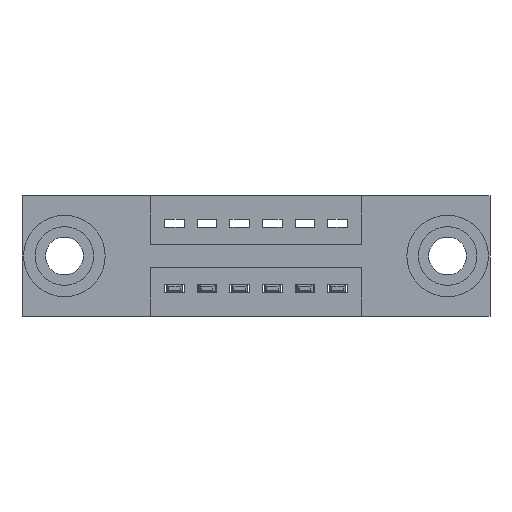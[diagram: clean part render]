
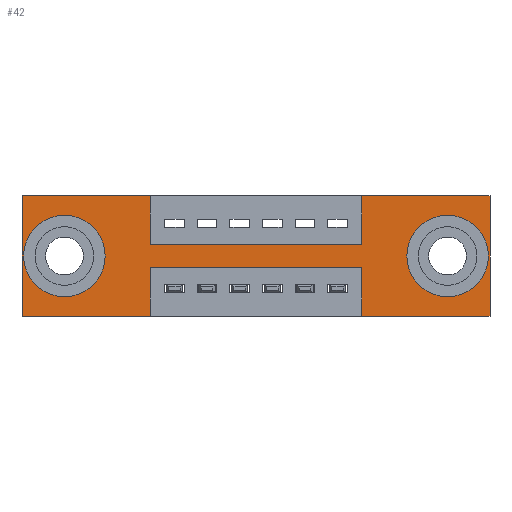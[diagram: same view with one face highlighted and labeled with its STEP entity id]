
A CAD part, front view. The second image highlights one B-rep face of the part: STEP entity #42.
In plain terms, the highlighted planar face has unit normal (0, -1, 0).
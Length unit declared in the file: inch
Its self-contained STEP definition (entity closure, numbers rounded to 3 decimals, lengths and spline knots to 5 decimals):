
#30 = LINE ( 'NONE', #667, #6235 ) ;
#42 = ADVANCED_FACE ( 'NONE', ( #6003, #6246, #522 ), #1607, .T. ) ;
#259 = CIRCLE ( 'NONE', #5577, 0.078 ) ;
#272 = LINE ( 'NONE', #1889, #1241 ) ;
#290 = VERTEX_POINT ( 'NONE', #9616 ) ;
#325 = EDGE_LOOP ( 'NONE', ( #2074, #9072 ) ) ;
#407 = EDGE_CURVE ( 'NONE', #9658, #2100, #30, .T. ) ;
#439 = EDGE_CURVE ( 'NONE', #6595, #7762, #1254, .T. ) ;
#522 = FACE_OUTER_BOUND ( 'NONE', #881, .T. ) ;
#655 = VERTEX_POINT ( 'NONE', #6087 ) ;
#667 = CARTESIAN_POINT ( 'NONE',  ( 0., 0., 0. ) ) ;
#716 = EDGE_CURVE ( 'NONE', #5456, #9203, #7302, .T. ) ;
#717 = DIRECTION ( 'NONE',  ( 0., 1., 0. ) ) ;
#740 = LINE ( 'NONE', #5035, #9411 ) ;
#802 = DIRECTION ( 'NONE',  ( 1., 0., 0. ) ) ;
#819 = EDGE_CURVE ( 'NONE', #8730, #6110, #9782, .T. ) ;
#852 = ORIENTED_EDGE ( 'NONE', *, *, #8790, .F. ) ;
#881 = EDGE_LOOP ( 'NONE', ( #1779, #3034, #2825, #911, #5724, #1565, #1600, #9178, #6298, #3192, #852, #7536 ) ) ;
#888 = EDGE_CURVE ( 'NONE', #9513, #8708, #272, .T. ) ;
#911 = ORIENTED_EDGE ( 'NONE', *, *, #2067, .F. ) ;
#1065 = DIRECTION ( 'NONE',  ( -1., 0., 0. ) ) ;
#1139 = EDGE_CURVE ( 'NONE', #1873, #8245, #8860, .T. ) ;
#1172 = EDGE_CURVE ( 'NONE', #4134, #6420, #259, .T. ) ;
#1241 = VECTOR ( 'NONE', #4912, 39.37008 ) ;
#1254 = LINE ( 'NONE', #5121, #1591 ) ;
#1565 = ORIENTED_EDGE ( 'NONE', *, *, #4197, .F. ) ;
#1591 = VECTOR ( 'NONE', #5888, 39.37008 ) ;
#1600 = ORIENTED_EDGE ( 'NONE', *, *, #4431, .F. ) ;
#1607 = PLANE ( 'NONE',  #7999 ) ;
#1616 = EDGE_CURVE ( 'NONE', #6420, #4134, #5499, .T. ) ;
#1639 = CARTESIAN_POINT ( 'NONE',  ( 0., 0., -0.37 ) ) ;
#1652 = DIRECTION ( 'NONE',  ( 0., 0., -1. ) ) ;
#1683 = LINE ( 'NONE', #1915, #2048 ) ;
#1717 = VECTOR ( 'NONE', #1652, 39.37008 ) ;
#1779 = ORIENTED_EDGE ( 'NONE', *, *, #716, .F. ) ;
#1873 = VERTEX_POINT ( 'NONE', #5526 ) ;
#1889 = CARTESIAN_POINT ( 'NONE',  ( 1.435, 0., 0. ) ) ;
#1915 = CARTESIAN_POINT ( 'NONE',  ( 0., 0., -0.37 ) ) ;
#1933 = CARTESIAN_POINT ( 'NONE',  ( 1.0425, 0., 0. ) ) ;
#1983 = ORIENTED_EDGE ( 'NONE', *, *, #1172, .T. ) ;
#2048 = VECTOR ( 'NONE', #1065, 39.37008 ) ;
#2067 = EDGE_CURVE ( 'NONE', #8708, #8730, #1683, .T. ) ;
#2074 = ORIENTED_EDGE ( 'NONE', *, *, #1139, .T. ) ;
#2100 = VERTEX_POINT ( 'NONE', #3443 ) ;
#2330 = DIRECTION ( 'NONE',  ( 0., 1., 0. ) ) ;
#2413 = DIRECTION ( 'NONE',  ( 0., 0., -1. ) ) ;
#2588 = DIRECTION ( 'NONE',  ( 0., 0., 1. ) ) ;
#2739 = DIRECTION ( 'NONE',  ( 0., 0., 1. ) ) ;
#2825 = ORIENTED_EDGE ( 'NONE', *, *, #819, .F. ) ;
#2883 = CARTESIAN_POINT ( 'NONE',  ( 0.13, 0., -0.185 ) ) ;
#3031 = DIRECTION ( 'NONE',  ( 0., 0., -1. ) ) ;
#3034 = ORIENTED_EDGE ( 'NONE', *, *, #7110, .F. ) ;
#3070 = VECTOR ( 'NONE', #2739, 39.37008 ) ;
#3192 = ORIENTED_EDGE ( 'NONE', *, *, #407, .F. ) ;
#3306 = CARTESIAN_POINT ( 'NONE',  ( 1.435, 0., -0.37 ) ) ;
#3443 = CARTESIAN_POINT ( 'NONE',  ( 0.3925, 0., 0. ) ) ;
#3511 = CARTESIAN_POINT ( 'NONE',  ( 1.0425, 0., -0.37 ) ) ;
#3578 = AXIS2_PLACEMENT_3D ( 'NONE', #2883, #7383, #8197 ) ;
#3701 = CARTESIAN_POINT ( 'NONE',  ( 0., 0., -0.37 ) ) ;
#3758 = CARTESIAN_POINT ( 'NONE',  ( 1.305, 0., -0.185 ) ) ;
#3828 = CARTESIAN_POINT ( 'NONE',  ( 0.3925, 0., -0.37 ) ) ;
#3847 = CARTESIAN_POINT ( 'NONE',  ( 0., 0., 0. ) ) ;
#3853 = CARTESIAN_POINT ( 'NONE',  ( 0., 0., 0. ) ) ;
#3937 = EDGE_CURVE ( 'NONE', #8245, #1873, #4155, .T. ) ;
#4005 = DIRECTION ( 'NONE',  ( 0., -1., 0. ) ) ;
#4048 = CARTESIAN_POINT ( 'NONE',  ( 0.13, 0., -0.263 ) ) ;
#4101 = LINE ( 'NONE', #5686, #1717 ) ;
#4134 = VERTEX_POINT ( 'NONE', #4391 ) ;
#4155 = CIRCLE ( 'NONE', #9719, 0.078 ) ;
#4197 = EDGE_CURVE ( 'NONE', #290, #9513, #4390, .T. ) ;
#4222 = CARTESIAN_POINT ( 'NONE',  ( 1.0425, 0., -0.15 ) ) ;
#4390 = LINE ( 'NONE', #3847, #6751 ) ;
#4391 = CARTESIAN_POINT ( 'NONE',  ( 0.13, 0., -0.107 ) ) ;
#4431 = EDGE_CURVE ( 'NONE', #7762, #290, #9601, .T. ) ;
#4768 = CARTESIAN_POINT ( 'NONE',  ( 1.305, 0., -0.263 ) ) ;
#4794 = DIRECTION ( 'NONE',  ( -1., 0., 0. ) ) ;
#4845 = DIRECTION ( 'NONE',  ( 0., 0., -1. ) ) ;
#4880 = CARTESIAN_POINT ( 'NONE',  ( 0.3925, 0., -0.37 ) ) ;
#4912 = DIRECTION ( 'NONE',  ( 0., 0., -1. ) ) ;
#4962 = CARTESIAN_POINT ( 'NONE',  ( 1.305, 0., -0.185 ) ) ;
#5035 = CARTESIAN_POINT ( 'NONE',  ( 0., 0., 0. ) ) ;
#5121 = CARTESIAN_POINT ( 'NONE',  ( 0.3925, 0., -0.15 ) ) ;
#5153 = DIRECTION ( 'NONE',  ( 1., 0., 0. ) ) ;
#5248 = CARTESIAN_POINT ( 'NONE',  ( 0.3925, 0., -0.22 ) ) ;
#5456 = VERTEX_POINT ( 'NONE', #5248 ) ;
#5499 = CIRCLE ( 'NONE', #3578, 0.078 ) ;
#5526 = CARTESIAN_POINT ( 'NONE',  ( 1.305, 0., -0.107 ) ) ;
#5577 = AXIS2_PLACEMENT_3D ( 'NONE', #9098, #2330, #7531 ) ;
#5686 = CARTESIAN_POINT ( 'NONE',  ( 0.3925, 0., 0. ) ) ;
#5724 = ORIENTED_EDGE ( 'NONE', *, *, #888, .F. ) ;
#5888 = DIRECTION ( 'NONE',  ( 1., 0., 0. ) ) ;
#6003 = FACE_BOUND ( 'NONE', #325, .T. ) ;
#6075 = AXIS2_PLACEMENT_3D ( 'NONE', #3758, #717, #3031 ) ;
#6087 = CARTESIAN_POINT ( 'NONE',  ( 0., 0., -0.37 ) ) ;
#6110 = VERTEX_POINT ( 'NONE', #7990 ) ;
#6235 = VECTOR ( 'NONE', #5153, 39.37008 ) ;
#6243 = LINE ( 'NONE', #6424, #6366 ) ;
#6246 = FACE_BOUND ( 'NONE', #6264, .T. ) ;
#6264 = EDGE_LOOP ( 'NONE', ( #1983, #7226 ) ) ;
#6298 = ORIENTED_EDGE ( 'NONE', *, *, #7425, .F. ) ;
#6366 = VECTOR ( 'NONE', #7160, 39.37008 ) ;
#6417 = CARTESIAN_POINT ( 'NONE',  ( 1.0425, 0., -0.37 ) ) ;
#6420 = VERTEX_POINT ( 'NONE', #4048 ) ;
#6424 = CARTESIAN_POINT ( 'NONE',  ( 0.3925, 0., -0.22 ) ) ;
#6595 = VERTEX_POINT ( 'NONE', #8884 ) ;
#6751 = VECTOR ( 'NONE', #802, 39.37008 ) ;
#7110 = EDGE_CURVE ( 'NONE', #6110, #5456, #6243, .T. ) ;
#7160 = DIRECTION ( 'NONE',  ( -1., 0., 0. ) ) ;
#7171 = VECTOR ( 'NONE', #4845, 39.37008 ) ;
#7226 = ORIENTED_EDGE ( 'NONE', *, *, #1616, .T. ) ;
#7302 = LINE ( 'NONE', #4880, #7171 ) ;
#7378 = EDGE_CURVE ( 'NONE', #9203, #655, #7902, .T. ) ;
#7383 = DIRECTION ( 'NONE',  ( 0., 1., 0. ) ) ;
#7406 = VECTOR ( 'NONE', #2588, 39.37008 ) ;
#7425 = EDGE_CURVE ( 'NONE', #2100, #6595, #4101, .T. ) ;
#7531 = DIRECTION ( 'NONE',  ( 0., 0., 1. ) ) ;
#7536 = ORIENTED_EDGE ( 'NONE', *, *, #7378, .F. ) ;
#7762 = VERTEX_POINT ( 'NONE', #4222 ) ;
#7902 = LINE ( 'NONE', #3701, #8745 ) ;
#7950 = DIRECTION ( 'NONE',  ( 0., 0., 1. ) ) ;
#7990 = CARTESIAN_POINT ( 'NONE',  ( 1.0425, 0., -0.22 ) ) ;
#7999 = AXIS2_PLACEMENT_3D ( 'NONE', #1639, #4005, #2413 ) ;
#8197 = DIRECTION ( 'NONE',  ( 0., 0., 1. ) ) ;
#8245 = VERTEX_POINT ( 'NONE', #4768 ) ;
#8574 = DIRECTION ( 'NONE',  ( 0., 1., 0. ) ) ;
#8708 = VERTEX_POINT ( 'NONE', #3306 ) ;
#8730 = VERTEX_POINT ( 'NONE', #3511 ) ;
#8745 = VECTOR ( 'NONE', #4794, 39.37008 ) ;
#8790 = EDGE_CURVE ( 'NONE', #655, #9658, #740, .T. ) ;
#8860 = CIRCLE ( 'NONE', #6075, 0.078 ) ;
#8884 = CARTESIAN_POINT ( 'NONE',  ( 0.3925, 0., -0.15 ) ) ;
#9072 = ORIENTED_EDGE ( 'NONE', *, *, #3937, .T. ) ;
#9098 = CARTESIAN_POINT ( 'NONE',  ( 0.13, 0., -0.185 ) ) ;
#9178 = ORIENTED_EDGE ( 'NONE', *, *, #439, .F. ) ;
#9203 = VERTEX_POINT ( 'NONE', #3828 ) ;
#9411 = VECTOR ( 'NONE', #7950, 39.37008 ) ;
#9513 = VERTEX_POINT ( 'NONE', #9740 ) ;
#9564 = DIRECTION ( 'NONE',  ( 0., 0., -1. ) ) ;
#9601 = LINE ( 'NONE', #1933, #3070 ) ;
#9616 = CARTESIAN_POINT ( 'NONE',  ( 1.0425, 0., 0. ) ) ;
#9658 = VERTEX_POINT ( 'NONE', #3853 ) ;
#9719 = AXIS2_PLACEMENT_3D ( 'NONE', #4962, #8574, #9564 ) ;
#9740 = CARTESIAN_POINT ( 'NONE',  ( 1.435, 0., 0. ) ) ;
#9782 = LINE ( 'NONE', #6417, #7406 ) ;
